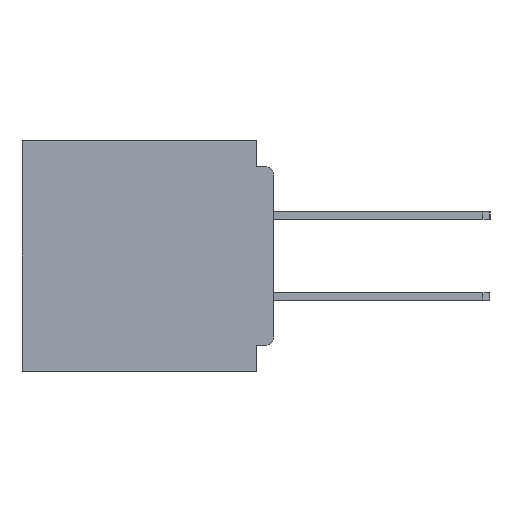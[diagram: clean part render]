
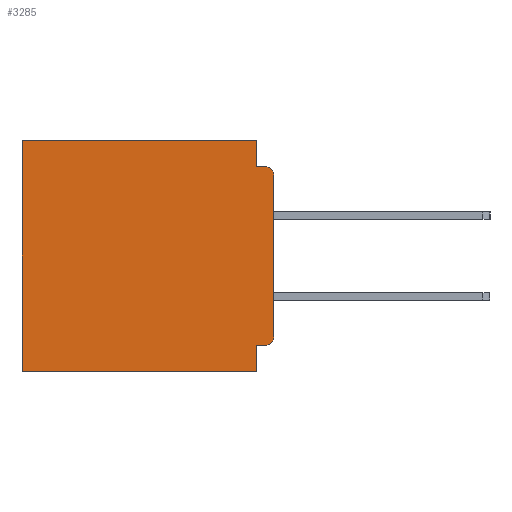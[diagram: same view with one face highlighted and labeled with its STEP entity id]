
A CAD part, left-side view. The second image highlights one B-rep face of the part: STEP entity #3285.
In plain terms, the highlighted planar face has unit normal (-1, 0, 0).
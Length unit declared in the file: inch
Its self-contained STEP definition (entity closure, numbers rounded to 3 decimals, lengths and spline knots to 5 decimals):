
#1222 = LINE ( 'NONE', #1458, #40229 ) ;
#1243 = CARTESIAN_POINT ( 'NONE',  ( 0.3, 0., -0.4 ) ) ;
#1284 = VERTEX_POINT ( 'NONE', #26164 ) ;
#1458 = CARTESIAN_POINT ( 'NONE',  ( 0.3, 0., -0.4 ) ) ;
#2379 = CARTESIAN_POINT ( 'NONE',  ( 0.3, 0., 0. ) ) ;
#3285 = ADVANCED_FACE ( 'NONE', ( #6854 ), #22515, .F. ) ;
#3547 = ORIENTED_EDGE ( 'NONE', *, *, #25064, .T. ) ;
#5999 = VECTOR ( 'NONE', #10336, 39.37008 ) ;
#6581 = AXIS2_PLACEMENT_3D ( 'NONE', #29395, #64597, #34455 ) ;
#6854 = FACE_OUTER_BOUND ( 'NONE', #46643, .T. ) ;
#7694 = VECTOR ( 'NONE', #39735, 39.37008 ) ;
#8998 = VERTEX_POINT ( 'NONE', #64981 ) ;
#9461 = DIRECTION ( 'NONE',  ( 0., 0., -1. ) ) ;
#9493 = EDGE_CURVE ( 'NONE', #41987, #27676, #38123, .T. ) ;
#9893 = DIRECTION ( 'NONE',  ( 1., 0., 0. ) ) ;
#9997 = VERTEX_POINT ( 'NONE', #57437 ) ;
#10248 = VECTOR ( 'NONE', #40511, 39.37008 ) ;
#10336 = DIRECTION ( 'NONE',  ( 0., 0., -1. ) ) ;
#11032 = CARTESIAN_POINT ( 'NONE',  ( 0.3, 0.031, 0. ) ) ;
#12368 = ORIENTED_EDGE ( 'NONE', *, *, #52369, .F. ) ;
#13251 = DIRECTION ( 'NONE',  ( 0., 0., -1. ) ) ;
#14887 = VERTEX_POINT ( 'NONE', #26203 ) ;
#16272 = ORIENTED_EDGE ( 'NONE', *, *, #18564, .F. ) ;
#18564 = EDGE_CURVE ( 'NONE', #56014, #20450, #19605, .T. ) ;
#19549 = ORIENTED_EDGE ( 'NONE', *, *, #9493, .F. ) ;
#19605 = LINE ( 'NONE', #61013, #5999 ) ;
#20450 = VERTEX_POINT ( 'NONE', #41455 ) ;
#22515 = PLANE ( 'NONE',  #59159 ) ;
#22943 = DIRECTION ( 'NONE',  ( -1., 0., 0. ) ) ;
#24282 = ORIENTED_EDGE ( 'NONE', *, *, #51271, .F. ) ;
#25064 = EDGE_CURVE ( 'NONE', #61971, #1284, #50591, .T. ) ;
#25190 = CARTESIAN_POINT ( 'NONE',  ( 0.3, 0., -0.06 ) ) ;
#25274 = CARTESIAN_POINT ( 'NONE',  ( 0.3, 0.437, -0.4 ) ) ;
#26164 = CARTESIAN_POINT ( 'NONE',  ( 0.3, 0.437, 0. ) ) ;
#26203 = CARTESIAN_POINT ( 'NONE',  ( 0.3, 0.015, -0.045 ) ) ;
#27266 = EDGE_CURVE ( 'NONE', #61971, #9997, #34944, .T. ) ;
#27676 = VERTEX_POINT ( 'NONE', #37210 ) ;
#29395 = CARTESIAN_POINT ( 'NONE',  ( 0.3, 0.015, -0.06 ) ) ;
#30465 = CARTESIAN_POINT ( 'NONE',  ( 0.3, 0.031, -0.355 ) ) ;
#31886 = AXIS2_PLACEMENT_3D ( 'NONE', #53213, #22943, #58276 ) ;
#34455 = DIRECTION ( 'NONE',  ( 0., 0., -1. ) ) ;
#34577 = ORIENTED_EDGE ( 'NONE', *, *, #41818, .T. ) ;
#34710 = EDGE_CURVE ( 'NONE', #1284, #54361, #54509, .T. ) ;
#34944 = LINE ( 'NONE', #43682, #58609 ) ;
#36550 = VECTOR ( 'NONE', #58169, 39.37008 ) ;
#37210 = CARTESIAN_POINT ( 'NONE',  ( 0.3, 0.031, -0.4 ) ) ;
#38118 = CARTESIAN_POINT ( 'NONE',  ( 0.3, 0.031, -0.4 ) ) ;
#38123 = LINE ( 'NONE', #38118, #36550 ) ;
#39735 = DIRECTION ( 'NONE',  ( 0., 1., 0. ) ) ;
#40229 = VECTOR ( 'NONE', #42190, 39.37008 ) ;
#40511 = DIRECTION ( 'NONE',  ( 0., -1., 0. ) ) ;
#40982 = ORIENTED_EDGE ( 'NONE', *, *, #53654, .T. ) ;
#41455 = CARTESIAN_POINT ( 'NONE',  ( 0.3, 0., -0.34 ) ) ;
#41818 = EDGE_CURVE ( 'NONE', #56014, #14887, #62644, .T. ) ;
#41987 = VERTEX_POINT ( 'NONE', #30465 ) ;
#42190 = DIRECTION ( 'NONE',  ( 0., 1., 0. ) ) ;
#43073 = DIRECTION ( 'NONE',  ( 0., 1., 0. ) ) ;
#43682 = CARTESIAN_POINT ( 'NONE',  ( 0.3, 0.031, 0. ) ) ;
#45584 = CARTESIAN_POINT ( 'NONE',  ( 0.3, 0., -0.045 ) ) ;
#46267 = EDGE_CURVE ( 'NONE', #27676, #54361, #1222, .T. ) ;
#46643 = EDGE_LOOP ( 'NONE', ( #16272, #34577, #24282, #55899, #3547, #57470, #56733, #19549, #12368, #40982 ) ) ;
#48179 = LINE ( 'NONE', #64774, #7694 ) ;
#49037 = VECTOR ( 'NONE', #43073, 39.37008 ) ;
#50238 = DIRECTION ( 'NONE',  ( 0., 0., -1. ) ) ;
#50591 = LINE ( 'NONE', #2379, #49037 ) ;
#51271 = EDGE_CURVE ( 'NONE', #9997, #14887, #64072, .T. ) ;
#52369 = EDGE_CURVE ( 'NONE', #8998, #41987, #48179, .T. ) ;
#53213 = CARTESIAN_POINT ( 'NONE',  ( 0.3, 0.015, -0.34 ) ) ;
#53654 = EDGE_CURVE ( 'NONE', #8998, #20450, #62930, .T. ) ;
#54361 = VERTEX_POINT ( 'NONE', #58847 ) ;
#54509 = LINE ( 'NONE', #25274, #64703 ) ;
#55899 = ORIENTED_EDGE ( 'NONE', *, *, #27266, .F. ) ;
#56014 = VERTEX_POINT ( 'NONE', #25190 ) ;
#56733 = ORIENTED_EDGE ( 'NONE', *, *, #46267, .F. ) ;
#57437 = CARTESIAN_POINT ( 'NONE',  ( 0.3, 0.031, -0.045 ) ) ;
#57470 = ORIENTED_EDGE ( 'NONE', *, *, #34710, .T. ) ;
#58169 = DIRECTION ( 'NONE',  ( 0., 0., -1. ) ) ;
#58276 = DIRECTION ( 'NONE',  ( 0., 0., -1. ) ) ;
#58609 = VECTOR ( 'NONE', #13251, 39.37008 ) ;
#58847 = CARTESIAN_POINT ( 'NONE',  ( 0.3, 0.437, -0.4 ) ) ;
#59159 = AXIS2_PLACEMENT_3D ( 'NONE', #1243, #9893, #9461 ) ;
#61013 = CARTESIAN_POINT ( 'NONE',  ( 0.3, 0., -0.4 ) ) ;
#61971 = VERTEX_POINT ( 'NONE', #11032 ) ;
#62644 = CIRCLE ( 'NONE', #6581, 0.015 ) ;
#62930 = CIRCLE ( 'NONE', #31886, 0.015 ) ;
#64072 = LINE ( 'NONE', #45584, #10248 ) ;
#64597 = DIRECTION ( 'NONE',  ( -1., 0., 0. ) ) ;
#64703 = VECTOR ( 'NONE', #50238, 39.37008 ) ;
#64774 = CARTESIAN_POINT ( 'NONE',  ( 0.3, 0., -0.355 ) ) ;
#64981 = CARTESIAN_POINT ( 'NONE',  ( 0.3, 0.015, -0.355 ) ) ;
